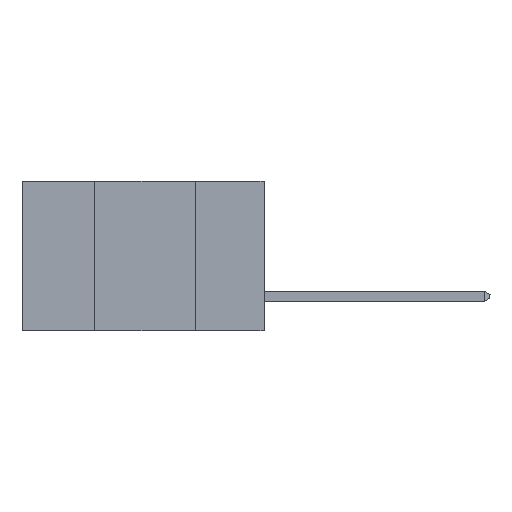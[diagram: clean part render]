
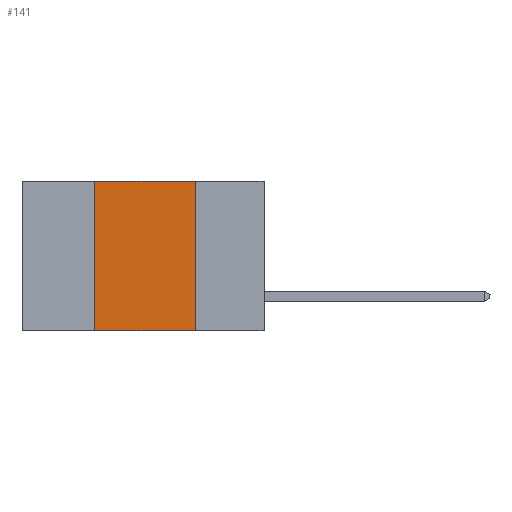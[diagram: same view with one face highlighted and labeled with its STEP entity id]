
A CAD part, left-side view. The second image highlights one B-rep face of the part: STEP entity #141.
In plain terms, the highlighted planar face has unit normal (-1, 0, 0).
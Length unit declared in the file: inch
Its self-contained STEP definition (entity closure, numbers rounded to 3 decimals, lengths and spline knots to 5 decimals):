
#141 = ADVANCED_FACE ( 'NONE', ( #4202 ), #9081, .F. ) ;
#213 = ORIENTED_EDGE ( 'NONE', *, *, #2574, .F. ) ;
#1098 = LINE ( 'NONE', #4312, #4032 ) ;
#1426 = CARTESIAN_POINT ( 'NONE',  ( 0., 0.17, -0.37 ) ) ;
#1904 = CARTESIAN_POINT ( 'NONE',  ( 0., 0.17, -0.37 ) ) ;
#1918 = CARTESIAN_POINT ( 'NONE',  ( 0., 0.42, 0. ) ) ;
#2095 = ORIENTED_EDGE ( 'NONE', *, *, #3302, .F. ) ;
#2446 = CARTESIAN_POINT ( 'NONE',  ( 0., 0.6, 0. ) ) ;
#2461 = ORIENTED_EDGE ( 'NONE', *, *, #9915, .F. ) ;
#2574 = EDGE_CURVE ( 'NONE', #5767, #4015, #5270, .T. ) ;
#2706 = DIRECTION ( 'NONE',  ( 0., -1., 0. ) ) ;
#3302 = EDGE_CURVE ( 'NONE', #10217, #5767, #1098, .T. ) ;
#3687 = EDGE_LOOP ( 'NONE', ( #213, #2095, #2461, #9106 ) ) ;
#3716 = EDGE_CURVE ( 'NONE', #9682, #4015, #9988, .T. ) ;
#4015 = VERTEX_POINT ( 'NONE', #1904 ) ;
#4032 = VECTOR ( 'NONE', #2706, 39.37008 ) ;
#4037 = VECTOR ( 'NONE', #4617, 39.37008 ) ;
#4147 = DIRECTION ( 'NONE',  ( 1., 0., 0. ) ) ;
#4202 = FACE_OUTER_BOUND ( 'NONE', #3687, .T. ) ;
#4312 = CARTESIAN_POINT ( 'NONE',  ( 0., 0.6, 0. ) ) ;
#4489 = DIRECTION ( 'NONE',  ( 0., 0., -1. ) ) ;
#4617 = DIRECTION ( 'NONE',  ( 0., 0., 1. ) ) ;
#5270 = LINE ( 'NONE', #1426, #10272 ) ;
#5767 = VERTEX_POINT ( 'NONE', #10210 ) ;
#6913 = CARTESIAN_POINT ( 'NONE',  ( 0., 0.42, -0.37 ) ) ;
#7542 = AXIS2_PLACEMENT_3D ( 'NONE', #2446, #4147, #8866 ) ;
#7802 = VECTOR ( 'NONE', #8432, 39.37008 ) ;
#8432 = DIRECTION ( 'NONE',  ( 0., -1., 0. ) ) ;
#8660 = LINE ( 'NONE', #9447, #4037 ) ;
#8866 = DIRECTION ( 'NONE',  ( 0., 0., -1. ) ) ;
#9081 = PLANE ( 'NONE',  #7542 ) ;
#9106 = ORIENTED_EDGE ( 'NONE', *, *, #3716, .T. ) ;
#9217 = CARTESIAN_POINT ( 'NONE',  ( 0., 0.6, -0.37 ) ) ;
#9447 = CARTESIAN_POINT ( 'NONE',  ( 0., 0.42, -0.37 ) ) ;
#9682 = VERTEX_POINT ( 'NONE', #6913 ) ;
#9915 = EDGE_CURVE ( 'NONE', #9682, #10217, #8660, .T. ) ;
#9988 = LINE ( 'NONE', #9217, #7802 ) ;
#10210 = CARTESIAN_POINT ( 'NONE',  ( 0., 0.17, 0. ) ) ;
#10217 = VERTEX_POINT ( 'NONE', #1918 ) ;
#10272 = VECTOR ( 'NONE', #4489, 39.37008 ) ;
